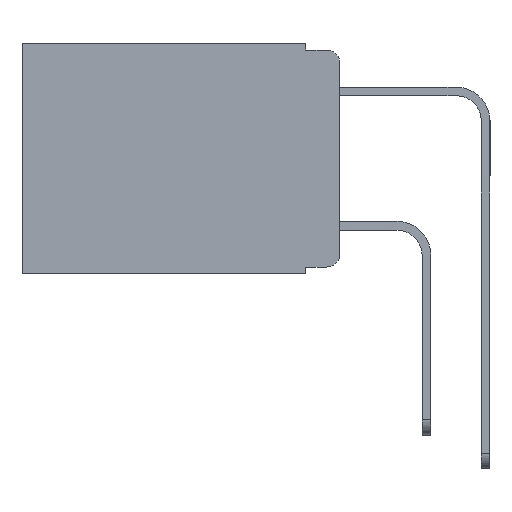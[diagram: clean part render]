
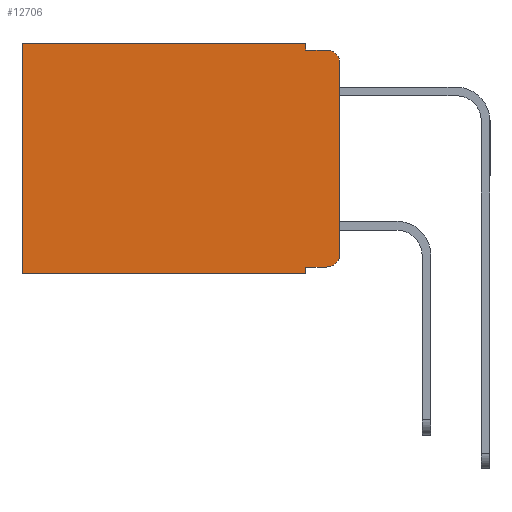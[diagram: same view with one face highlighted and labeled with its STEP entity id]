
A CAD part, left-side view. The second image highlights one B-rep face of the part: STEP entity #12706.
In plain terms, the highlighted planar face has unit normal (-1, 0, 0).
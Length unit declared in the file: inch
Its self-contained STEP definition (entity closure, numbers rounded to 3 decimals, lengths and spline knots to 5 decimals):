
#141 = ORIENTED_EDGE ( 'NONE', *, *, #1615, .T. ) ;
#167 = ORIENTED_EDGE ( 'NONE', *, *, #11363, .F. ) ;
#420 = DIRECTION ( 'NONE',  ( 0., 0., -1. ) ) ;
#532 = VECTOR ( 'NONE', #5946, 39.37008 ) ;
#1071 = LINE ( 'NONE', #5793, #13041 ) ;
#1519 = CARTESIAN_POINT ( 'NONE',  ( 0.298, 0., -0.313 ) ) ;
#1615 = EDGE_CURVE ( 'NONE', #6744, #4494, #3867, .T. ) ;
#1664 = VERTEX_POINT ( 'NONE', #14467 ) ;
#1704 = EDGE_CURVE ( 'NONE', #14132, #11214, #11552, .T. ) ;
#1842 = VECTOR ( 'NONE', #6837, 39.37008 ) ;
#2194 = DIRECTION ( 'NONE',  ( 0., -1., 0. ) ) ;
#2254 = CARTESIAN_POINT ( 'NONE',  ( 0.298, 0.051, 0. ) ) ;
#2762 = CARTESIAN_POINT ( 'NONE',  ( 0.298, 0.02, -0.313 ) ) ;
#2840 = EDGE_CURVE ( 'NONE', #10754, #6548, #15028, .T. ) ;
#2954 = CARTESIAN_POINT ( 'NONE',  ( 0.298, 0., -0.03 ) ) ;
#3120 = ORIENTED_EDGE ( 'NONE', *, *, #12077, .F. ) ;
#3140 = CARTESIAN_POINT ( 'NONE',  ( 0.298, 0.051, -0.333 ) ) ;
#3180 = DIRECTION ( 'NONE',  ( 0., 0., -1. ) ) ;
#3240 = LINE ( 'NONE', #7829, #6403 ) ;
#3486 = ORIENTED_EDGE ( 'NONE', *, *, #1704, .F. ) ;
#3867 = LINE ( 'NONE', #13755, #532 ) ;
#4009 = DIRECTION ( 'NONE',  ( 0., 0., -1. ) ) ;
#4075 = VECTOR ( 'NONE', #6910, 39.37008 ) ;
#4161 = FACE_OUTER_BOUND ( 'NONE', #7443, .T. ) ;
#4355 = ORIENTED_EDGE ( 'NONE', *, *, #12990, .T. ) ;
#4474 = EDGE_CURVE ( 'NONE', #4494, #10829, #5069, .T. ) ;
#4494 = VERTEX_POINT ( 'NONE', #13520 ) ;
#4828 = ORIENTED_EDGE ( 'NONE', *, *, #2840, .F. ) ;
#4887 = CARTESIAN_POINT ( 'NONE',  ( 0.298, 0.02, -0.333 ) ) ;
#5069 = LINE ( 'NONE', #12763, #1842 ) ;
#5683 = VECTOR ( 'NONE', #14454, 39.37008 ) ;
#5793 = CARTESIAN_POINT ( 'NONE',  ( 0.298, 0.051, -0.01 ) ) ;
#5826 = CARTESIAN_POINT ( 'NONE',  ( 0.298, 0., 0. ) ) ;
#5910 = VERTEX_POINT ( 'NONE', #14447 ) ;
#5938 = EDGE_CURVE ( 'NONE', #10754, #12856, #9241, .T. ) ;
#5946 = DIRECTION ( 'NONE',  ( 0., 1., 0. ) ) ;
#6133 = VECTOR ( 'NONE', #14589, 39.37008 ) ;
#6403 = VECTOR ( 'NONE', #11126, 39.37008 ) ;
#6548 = VERTEX_POINT ( 'NONE', #10122 ) ;
#6744 = VERTEX_POINT ( 'NONE', #11726 ) ;
#6837 = DIRECTION ( 'NONE',  ( 0., 0., -1. ) ) ;
#6910 = DIRECTION ( 'NONE',  ( 0., 1., 0. ) ) ;
#6999 = DIRECTION ( 'NONE',  ( 1., 0., 0. ) ) ;
#7198 = EDGE_CURVE ( 'NONE', #6548, #10829, #13118, .T. ) ;
#7443 = EDGE_LOOP ( 'NONE', ( #3486, #12434, #3120, #167, #141, #14692, #9183, #4828, #12942, #4355 ) ) ;
#7721 = DIRECTION ( 'NONE',  ( -1., 0., 0. ) ) ;
#7829 = CARTESIAN_POINT ( 'NONE',  ( 0.298, 0.051, 0. ) ) ;
#7890 = CARTESIAN_POINT ( 'NONE',  ( 0.298, 0.473, -0.343 ) ) ;
#8812 = AXIS2_PLACEMENT_3D ( 'NONE', #14376, #7721, #420 ) ;
#9183 = ORIENTED_EDGE ( 'NONE', *, *, #7198, .F. ) ;
#9241 = LINE ( 'NONE', #3140, #6133 ) ;
#10122 = CARTESIAN_POINT ( 'NONE',  ( 0.298, 0.051, -0.343 ) ) ;
#10754 = VERTEX_POINT ( 'NONE', #14406 ) ;
#10829 = VERTEX_POINT ( 'NONE', #7890 ) ;
#10838 = AXIS2_PLACEMENT_3D ( 'NONE', #2762, #10902, #4009 ) ;
#10902 = DIRECTION ( 'NONE',  ( -1., 0., 0. ) ) ;
#11126 = DIRECTION ( 'NONE',  ( 0., 0., -1. ) ) ;
#11214 = VERTEX_POINT ( 'NONE', #1519 ) ;
#11220 = VECTOR ( 'NONE', #3180, 39.37008 ) ;
#11363 = EDGE_CURVE ( 'NONE', #6744, #5910, #3240, .T. ) ;
#11429 = CARTESIAN_POINT ( 'NONE',  ( 0.298, 0., -0.343 ) ) ;
#11552 = LINE ( 'NONE', #12105, #11220 ) ;
#11726 = CARTESIAN_POINT ( 'NONE',  ( 0.298, 0.051, 0. ) ) ;
#12077 = EDGE_CURVE ( 'NONE', #5910, #1664, #1071, .T. ) ;
#12105 = CARTESIAN_POINT ( 'NONE',  ( 0.298, 0., 0. ) ) ;
#12434 = ORIENTED_EDGE ( 'NONE', *, *, #13576, .T. ) ;
#12471 = CIRCLE ( 'NONE', #8812, 0.02 ) ;
#12536 = AXIS2_PLACEMENT_3D ( 'NONE', #5826, #6999, #14836 ) ;
#12550 = PLANE ( 'NONE',  #12536 ) ;
#12706 = ADVANCED_FACE ( 'NONE', ( #4161 ), #12550, .F. ) ;
#12763 = CARTESIAN_POINT ( 'NONE',  ( 0.298, 0.473, 0. ) ) ;
#12856 = VERTEX_POINT ( 'NONE', #4887 ) ;
#12942 = ORIENTED_EDGE ( 'NONE', *, *, #5938, .T. ) ;
#12990 = EDGE_CURVE ( 'NONE', #12856, #11214, #14971, .T. ) ;
#13041 = VECTOR ( 'NONE', #2194, 39.37008 ) ;
#13118 = LINE ( 'NONE', #11429, #4075 ) ;
#13520 = CARTESIAN_POINT ( 'NONE',  ( 0.298, 0.473, 0. ) ) ;
#13576 = EDGE_CURVE ( 'NONE', #14132, #1664, #12471, .T. ) ;
#13755 = CARTESIAN_POINT ( 'NONE',  ( 0.298, 0., 0. ) ) ;
#14132 = VERTEX_POINT ( 'NONE', #2954 ) ;
#14376 = CARTESIAN_POINT ( 'NONE',  ( 0.298, 0.02, -0.03 ) ) ;
#14406 = CARTESIAN_POINT ( 'NONE',  ( 0.298, 0.051, -0.333 ) ) ;
#14447 = CARTESIAN_POINT ( 'NONE',  ( 0.298, 0.051, -0.01 ) ) ;
#14454 = DIRECTION ( 'NONE',  ( 0., 0., -1. ) ) ;
#14467 = CARTESIAN_POINT ( 'NONE',  ( 0.298, 0.02, -0.01 ) ) ;
#14589 = DIRECTION ( 'NONE',  ( 0., -1., 0. ) ) ;
#14692 = ORIENTED_EDGE ( 'NONE', *, *, #4474, .T. ) ;
#14836 = DIRECTION ( 'NONE',  ( 0., 0., -1. ) ) ;
#14971 = CIRCLE ( 'NONE', #10838, 0.02 ) ;
#15028 = LINE ( 'NONE', #2254, #5683 ) ;
